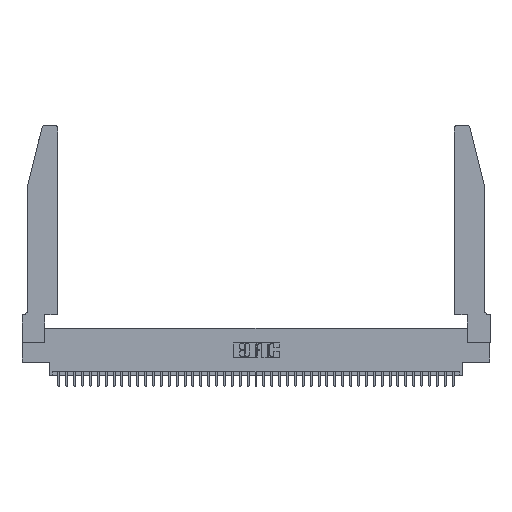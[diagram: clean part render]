
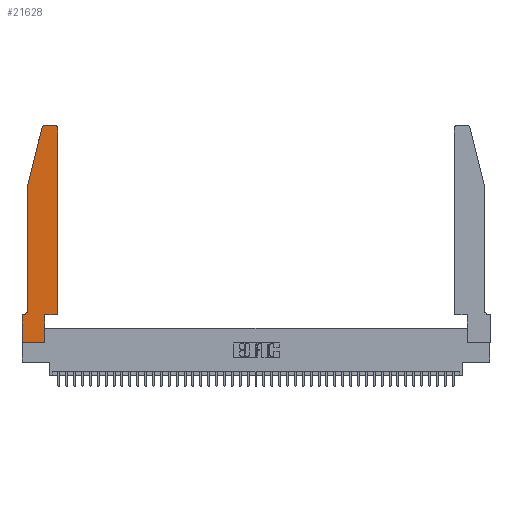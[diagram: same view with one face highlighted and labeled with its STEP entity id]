
A CAD part, top view. The second image highlights one B-rep face of the part: STEP entity #21628.
In plain terms, the highlighted planar face has unit normal (0, 0, 1).
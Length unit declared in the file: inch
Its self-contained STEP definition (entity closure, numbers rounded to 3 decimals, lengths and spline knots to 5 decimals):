
#206 = LINE ( 'NONE', #19944, #30419 ) ;
#281 = DIRECTION ( 'NONE',  ( -1., 0., 0. ) ) ;
#288 = CIRCLE ( 'NONE', #18200, 0.07 ) ;
#803 = VERTEX_POINT ( 'NONE', #23417 ) ;
#1648 = FACE_OUTER_BOUND ( 'NONE', #34253, .T. ) ;
#2401 = CARTESIAN_POINT ( 'NONE',  ( 0., 0.35, 0.37 ) ) ;
#2566 = DIRECTION ( 'NONE',  ( 0., 0., 1. ) ) ;
#2626 = CARTESIAN_POINT ( 'NONE',  ( 0.4505, 0.35, 0.37 ) ) ;
#2698 = VECTOR ( 'NONE', #12717, 39.37008 ) ;
#3186 = EDGE_CURVE ( 'NONE', #22621, #34708, #32531, .T. ) ;
#3944 = DIRECTION ( 'NONE',  ( 1., 0., 0. ) ) ;
#4019 = ORIENTED_EDGE ( 'NONE', *, *, #4268, .T. ) ;
#4268 = EDGE_CURVE ( 'NONE', #14907, #28259, #27157, .T. ) ;
#5116 = ORIENTED_EDGE ( 'NONE', *, *, #35349, .T. ) ;
#5195 = AXIS2_PLACEMENT_3D ( 'NONE', #33332, #2566, #12799 ) ;
#5249 = ORIENTED_EDGE ( 'NONE', *, *, #26460, .T. ) ;
#6996 = LINE ( 'NONE', #30962, #35616 ) ;
#9288 = CARTESIAN_POINT ( 'NONE',  ( 0.0755, 0.35, 0.37 ) ) ;
#9637 = CARTESIAN_POINT ( 'NONE',  ( 0.0755, 2., 0.37 ) ) ;
#9879 = VERTEX_POINT ( 'NONE', #2401 ) ;
#10328 = CARTESIAN_POINT ( 'NONE',  ( 0.284, 2.75, 0.37 ) ) ;
#10343 = VECTOR ( 'NONE', #31845, 39.37008 ) ;
#10366 = CARTESIAN_POINT ( 'NONE',  ( 0.2865, 0.35, 0.37 ) ) ;
#10368 = ORIENTED_EDGE ( 'NONE', *, *, #42420, .T. ) ;
#10673 = VECTOR ( 'NONE', #42726, 39.37008 ) ;
#10726 = EDGE_CURVE ( 'NONE', #13763, #803, #288, .T. ) ;
#11063 = VERTEX_POINT ( 'NONE', #35882 ) ;
#12024 = CARTESIAN_POINT ( 'NONE',  ( 0.2605, 2.75, 0.37 ) ) ;
#12717 = DIRECTION ( 'NONE',  ( -0.239, -0.971, 0. ) ) ;
#12799 = DIRECTION ( 'NONE',  ( 1., 0., 0. ) ) ;
#13092 = CARTESIAN_POINT ( 'NONE',  ( 0.284, 2.72, 0.37 ) ) ;
#13763 = VERTEX_POINT ( 'NONE', #29252 ) ;
#13838 = CARTESIAN_POINT ( 'NONE',  ( 0.2865, 0.35, 0.37 ) ) ;
#14134 = DIRECTION ( 'NONE',  ( 1., 0., 0. ) ) ;
#14907 = VERTEX_POINT ( 'NONE', #10366 ) ;
#15019 = EDGE_CURVE ( 'NONE', #28099, #11063, #206, .T. ) ;
#15451 = VECTOR ( 'NONE', #36878, 39.37008 ) ;
#16062 = CARTESIAN_POINT ( 'NONE',  ( 0.25487, 2.72718, 0.37 ) ) ;
#16634 = EDGE_CURVE ( 'NONE', #11063, #14907, #29231, .T. ) ;
#17039 = EDGE_CURVE ( 'NONE', #34523, #31638, #21238, .T. ) ;
#18200 = AXIS2_PLACEMENT_3D ( 'NONE', #37355, #20559, #281 ) ;
#19126 = DIRECTION ( 'NONE',  ( 0., 0., 1. ) ) ;
#19944 = CARTESIAN_POINT ( 'NONE',  ( 0., 0., 0.37 ) ) ;
#20285 = VECTOR ( 'NONE', #26197, 39.37008 ) ;
#20559 = DIRECTION ( 'NONE',  ( 0., 0., -1. ) ) ;
#20882 = AXIS2_PLACEMENT_3D ( 'NONE', #25537, #19126, #32258 ) ;
#21238 = LINE ( 'NONE', #36772, #2698 ) ;
#21291 = EDGE_CURVE ( 'NONE', #34708, #29718, #38142, .T. ) ;
#21628 = ADVANCED_FACE ( 'NONE', ( #1648 ), #29965, .T. ) ;
#22417 = ORIENTED_EDGE ( 'NONE', *, *, #17039, .T. ) ;
#22621 = VERTEX_POINT ( 'NONE', #26140 ) ;
#22978 = ORIENTED_EDGE ( 'NONE', *, *, #3186, .T. ) ;
#23235 = DIRECTION ( 'NONE',  ( -1., 0., 0. ) ) ;
#23417 = CARTESIAN_POINT ( 'NONE',  ( 0.0055, 0.35, 0.37 ) ) ;
#23509 = DIRECTION ( 'NONE',  ( 0., -1., 0. ) ) ;
#23641 = LINE ( 'NONE', #42436, #10343 ) ;
#24330 = DIRECTION ( 'NONE',  ( 0., 1., 0. ) ) ;
#25405 = EDGE_CURVE ( 'NONE', #803, #9879, #37302, .T. ) ;
#25537 = CARTESIAN_POINT ( 'NONE',  ( 0.4205, 2.72, 0.37 ) ) ;
#26140 = CARTESIAN_POINT ( 'NONE',  ( 0.4505, 2.72, 0.37 ) ) ;
#26197 = DIRECTION ( 'NONE',  ( 1., 0., 0. ) ) ;
#26460 = EDGE_CURVE ( 'NONE', #9879, #28099, #23641, .T. ) ;
#27157 = LINE ( 'NONE', #2626, #20285 ) ;
#28099 = VERTEX_POINT ( 'NONE', #35439 ) ;
#28259 = VERTEX_POINT ( 'NONE', #39120 ) ;
#29006 = ORIENTED_EDGE ( 'NONE', *, *, #15019, .T. ) ;
#29231 = LINE ( 'NONE', #13838, #15451 ) ;
#29252 = CARTESIAN_POINT ( 'NONE',  ( 0.0755, 0.42, 0.37 ) ) ;
#29557 = AXIS2_PLACEMENT_3D ( 'NONE', #13092, #30990, #14134 ) ;
#29718 = VERTEX_POINT ( 'NONE', #10328 ) ;
#29965 = PLANE ( 'NONE',  #5195 ) ;
#30419 = VECTOR ( 'NONE', #3944, 39.37008 ) ;
#30962 = CARTESIAN_POINT ( 'NONE',  ( 0.4505, 0.35, 0.37 ) ) ;
#30990 = DIRECTION ( 'NONE',  ( 0., 0., 1. ) ) ;
#31227 = EDGE_CURVE ( 'NONE', #29718, #34523, #38720, .T. ) ;
#31638 = VERTEX_POINT ( 'NONE', #9637 ) ;
#31845 = DIRECTION ( 'NONE',  ( 0., -1., 0. ) ) ;
#32258 = DIRECTION ( 'NONE',  ( 1., 0., 0. ) ) ;
#32531 = CIRCLE ( 'NONE', #20882, 0.03 ) ;
#32596 = VECTOR ( 'NONE', #23235, 39.37008 ) ;
#33238 = ORIENTED_EDGE ( 'NONE', *, *, #10726, .T. ) ;
#33332 = CARTESIAN_POINT ( 'NONE',  ( 0., 0.35, 0.37 ) ) ;
#34253 = EDGE_LOOP ( 'NONE', ( #39967, #41957, #22417, #10368, #33238, #40328, #5249, #29006, #35729, #4019, #5116, #22978 ) ) ;
#34523 = VERTEX_POINT ( 'NONE', #16062 ) ;
#34708 = VERTEX_POINT ( 'NONE', #34964 ) ;
#34964 = CARTESIAN_POINT ( 'NONE',  ( 0.4205, 2.75, 0.37 ) ) ;
#35349 = EDGE_CURVE ( 'NONE', #28259, #22621, #6996, .T. ) ;
#35439 = CARTESIAN_POINT ( 'NONE',  ( 0., 0., 0.37 ) ) ;
#35616 = VECTOR ( 'NONE', #24330, 39.37008 ) ;
#35660 = VECTOR ( 'NONE', #23509, 39.37008 ) ;
#35729 = ORIENTED_EDGE ( 'NONE', *, *, #16634, .T. ) ;
#35882 = CARTESIAN_POINT ( 'NONE',  ( 0.2865, 0., 0.37 ) ) ;
#36758 = CARTESIAN_POINT ( 'NONE',  ( 0.0755, 2., 0.37 ) ) ;
#36772 = CARTESIAN_POINT ( 'NONE',  ( 0.0755, 2., 0.37 ) ) ;
#36878 = DIRECTION ( 'NONE',  ( 0., 1., 0. ) ) ;
#37302 = LINE ( 'NONE', #9288, #32596 ) ;
#37355 = CARTESIAN_POINT ( 'NONE',  ( 0.0055, 0.42, 0.37 ) ) ;
#38142 = LINE ( 'NONE', #12024, #10673 ) ;
#38720 = CIRCLE ( 'NONE', #29557, 0.03 ) ;
#39120 = CARTESIAN_POINT ( 'NONE',  ( 0.4505, 0.35, 0.37 ) ) ;
#39967 = ORIENTED_EDGE ( 'NONE', *, *, #21291, .T. ) ;
#40328 = ORIENTED_EDGE ( 'NONE', *, *, #25405, .T. ) ;
#41957 = ORIENTED_EDGE ( 'NONE', *, *, #31227, .T. ) ;
#42420 = EDGE_CURVE ( 'NONE', #31638, #13763, #43035, .T. ) ;
#42436 = CARTESIAN_POINT ( 'NONE',  ( 0., 0., 0.37 ) ) ;
#42726 = DIRECTION ( 'NONE',  ( -1., 0., 0. ) ) ;
#43035 = LINE ( 'NONE', #36758, #35660 ) ;
